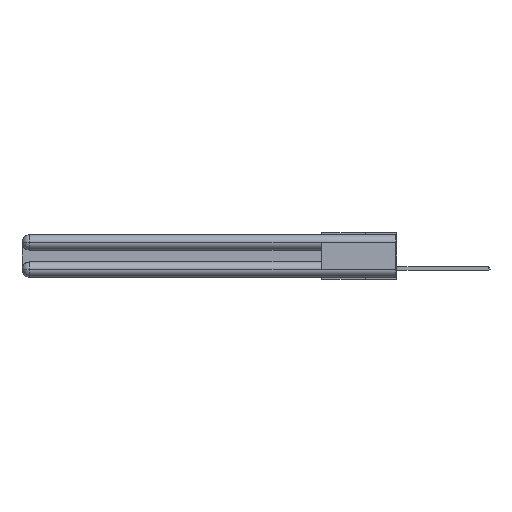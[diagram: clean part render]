
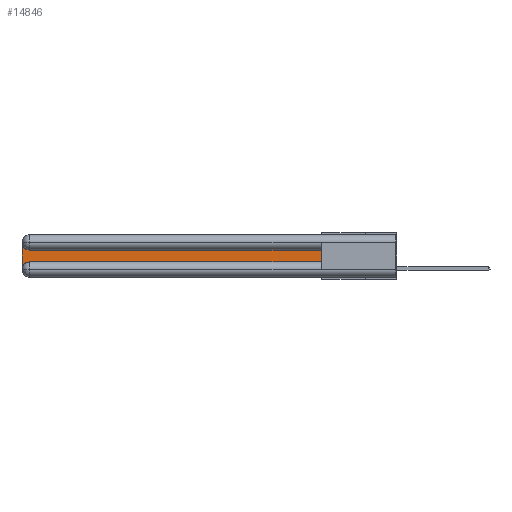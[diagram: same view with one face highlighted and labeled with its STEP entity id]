
A CAD part, left-side view. The second image highlights one B-rep face of the part: STEP entity #14846.
In plain terms, the highlighted planar face has unit normal (-1, 0, 0).
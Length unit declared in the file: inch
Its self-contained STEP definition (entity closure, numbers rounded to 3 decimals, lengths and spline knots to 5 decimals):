
#420 = ORIENTED_EDGE ( 'NONE', *, *, #9940, .T. ) ;
#1259 = CARTESIAN_POINT ( 'NONE',  ( 0.075, 0.6, -0.2175 ) ) ;
#1653 = DIRECTION ( 'NONE',  ( 1., 0., 0. ) ) ;
#1939 = EDGE_CURVE ( 'NONE', #16125, #29498, #2184, .T. ) ;
#2124 = LINE ( 'NONE', #1259, #8256 ) ;
#2184 = LINE ( 'NONE', #8126, #5431 ) ;
#2576 = CARTESIAN_POINT ( 'NONE',  ( 0.075, 2.94, -0.2175 ) ) ;
#2685 = CARTESIAN_POINT ( 'NONE',  ( 0.075, 2.94, -0.1225 ) ) ;
#2903 = ORIENTED_EDGE ( 'NONE', *, *, #1939, .T. ) ;
#3265 = EDGE_CURVE ( 'NONE', #24384, #12232, #29580, .T. ) ;
#3964 = CARTESIAN_POINT ( 'NONE',  ( 0.075, 2.94, -0.2775 ) ) ;
#4966 = AXIS2_PLACEMENT_3D ( 'NONE', #14804, #10011, #9908 ) ;
#5431 = VECTOR ( 'NONE', #18062, 39.37008 ) ;
#5503 = CARTESIAN_POINT ( 'NONE',  ( 0.075, 0.6, -0.1225 ) ) ;
#5866 = EDGE_CURVE ( 'NONE', #29498, #22639, #24298, .T. ) ;
#8126 = CARTESIAN_POINT ( 'NONE',  ( 0.075, 0.6, -0.2175 ) ) ;
#8256 = VECTOR ( 'NONE', #19638, 39.37008 ) ;
#9155 = CARTESIAN_POINT ( 'NONE',  ( 0.075, 3., -0.2175 ) ) ;
#9590 = DIRECTION ( 'NONE',  ( 1., 0., 0. ) ) ;
#9908 = DIRECTION ( 'NONE',  ( 0., 0., -1. ) ) ;
#9940 = EDGE_CURVE ( 'NONE', #12232, #20522, #12998, .T. ) ;
#9999 = VECTOR ( 'NONE', #20403, 39.37008 ) ;
#10011 = DIRECTION ( 'NONE',  ( 1., 0., 0. ) ) ;
#10484 = ORIENTED_EDGE ( 'NONE', *, *, #26613, .T. ) ;
#10726 = AXIS2_PLACEMENT_3D ( 'NONE', #3964, #1653, #26662 ) ;
#11295 = EDGE_CURVE ( 'NONE', #22639, #24384, #26679, .T. ) ;
#11824 = CARTESIAN_POINT ( 'NONE',  ( 0.075, 3., -0.0625 ) ) ;
#12232 = VERTEX_POINT ( 'NONE', #22474 ) ;
#12998 = CIRCLE ( 'NONE', #10726, 0.06 ) ;
#14710 = VECTOR ( 'NONE', #29111, 39.37008 ) ;
#14804 = CARTESIAN_POINT ( 'NONE',  ( 0.075, 2.94, -0.0625 ) ) ;
#14846 = ADVANCED_FACE ( 'NONE', ( #24852 ), #23203, .F. ) ;
#16081 = CARTESIAN_POINT ( 'NONE',  ( 0.075, 0.6, -0.1225 ) ) ;
#16125 = VERTEX_POINT ( 'NONE', #23034 ) ;
#18062 = DIRECTION ( 'NONE',  ( 0., 0., 1. ) ) ;
#19576 = AXIS2_PLACEMENT_3D ( 'NONE', #27993, #9590, #25490 ) ;
#19638 = DIRECTION ( 'NONE',  ( 0., -1., 0. ) ) ;
#20403 = DIRECTION ( 'NONE',  ( 0., 0., -1. ) ) ;
#20522 = VERTEX_POINT ( 'NONE', #2576 ) ;
#22474 = CARTESIAN_POINT ( 'NONE',  ( 0.075, 3., -0.2775 ) ) ;
#22639 = VERTEX_POINT ( 'NONE', #2685 ) ;
#23034 = CARTESIAN_POINT ( 'NONE',  ( 0.075, 0.6, -0.2175 ) ) ;
#23203 = PLANE ( 'NONE',  #19576 ) ;
#24146 = ORIENTED_EDGE ( 'NONE', *, *, #11295, .T. ) ;
#24298 = LINE ( 'NONE', #5503, #14710 ) ;
#24384 = VERTEX_POINT ( 'NONE', #11824 ) ;
#24606 = ORIENTED_EDGE ( 'NONE', *, *, #3265, .T. ) ;
#24852 = FACE_OUTER_BOUND ( 'NONE', #29473, .T. ) ;
#25490 = DIRECTION ( 'NONE',  ( 0., 0., -1. ) ) ;
#26613 = EDGE_CURVE ( 'NONE', #20522, #16125, #2124, .T. ) ;
#26662 = DIRECTION ( 'NONE',  ( 0., 0., -1. ) ) ;
#26679 = CIRCLE ( 'NONE', #4966, 0.06 ) ;
#27993 = CARTESIAN_POINT ( 'NONE',  ( 0.075, 3., -0.1225 ) ) ;
#28849 = ORIENTED_EDGE ( 'NONE', *, *, #5866, .T. ) ;
#29111 = DIRECTION ( 'NONE',  ( 0., 1., 0. ) ) ;
#29473 = EDGE_LOOP ( 'NONE', ( #28849, #24146, #24606, #420, #10484, #2903 ) ) ;
#29498 = VERTEX_POINT ( 'NONE', #16081 ) ;
#29580 = LINE ( 'NONE', #9155, #9999 ) ;
